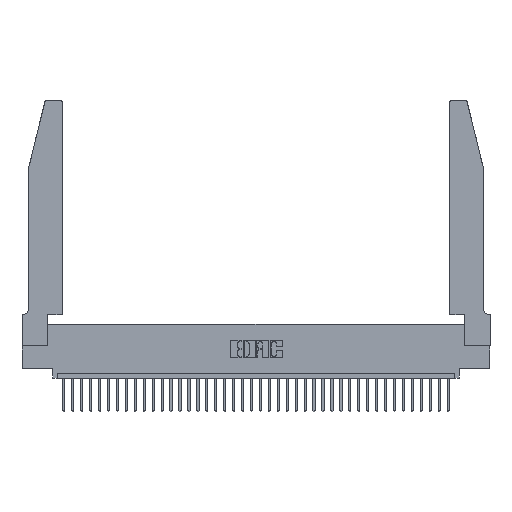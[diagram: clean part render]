
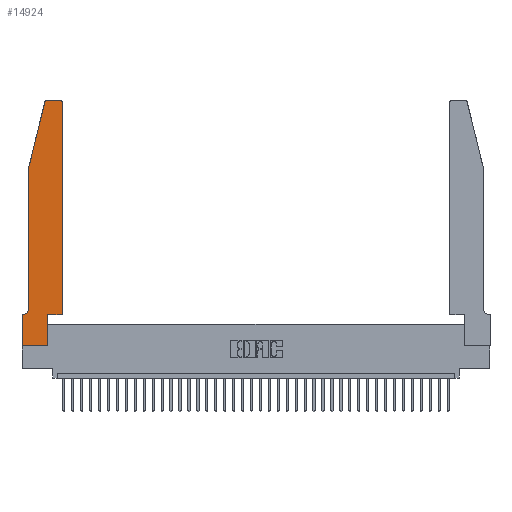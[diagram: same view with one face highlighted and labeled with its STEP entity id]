
A CAD part, top view. The second image highlights one B-rep face of the part: STEP entity #14924.
In plain terms, the highlighted planar face has unit normal (0, 0, 1).
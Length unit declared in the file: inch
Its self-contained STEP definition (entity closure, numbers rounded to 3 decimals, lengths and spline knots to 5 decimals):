
#1022 = ORIENTED_EDGE ( 'NONE', *, *, #9327, .T. ) ;
#1280 = AXIS2_PLACEMENT_3D ( 'NONE', #3978, #37201, #30963 ) ;
#2041 = LINE ( 'NONE', #30785, #21114 ) ;
#2487 = DIRECTION ( 'NONE',  ( -1., 0., 0. ) ) ;
#2624 = CARTESIAN_POINT ( 'NONE',  ( 0.284, 2.75, 0.37 ) ) ;
#2800 = DIRECTION ( 'NONE',  ( 1., 0., 0. ) ) ;
#3412 = CARTESIAN_POINT ( 'NONE',  ( 0.4505, 0.35, 0.37 ) ) ;
#3474 = AXIS2_PLACEMENT_3D ( 'NONE', #17169, #36990, #7970 ) ;
#3978 = CARTESIAN_POINT ( 'NONE',  ( 0.284, 2.72, 0.37 ) ) ;
#4354 = CARTESIAN_POINT ( 'NONE',  ( 0.4505, 0.35, 0.37 ) ) ;
#4564 = VERTEX_POINT ( 'NONE', #9132 ) ;
#4585 = ORIENTED_EDGE ( 'NONE', *, *, #28018, .T. ) ;
#5076 = DIRECTION ( 'NONE',  ( 0., -1., 0. ) ) ;
#5438 = EDGE_CURVE ( 'NONE', #6268, #27754, #9279, .T. ) ;
#5701 = EDGE_CURVE ( 'NONE', #22428, #12500, #17508, .T. ) ;
#5960 = VERTEX_POINT ( 'NONE', #11096 ) ;
#6268 = VERTEX_POINT ( 'NONE', #3412 ) ;
#6468 = ORIENTED_EDGE ( 'NONE', *, *, #10294, .T. ) ;
#6600 = FACE_OUTER_BOUND ( 'NONE', #17381, .T. ) ;
#7970 = DIRECTION ( 'NONE',  ( -1., 0., 0. ) ) ;
#8571 = CARTESIAN_POINT ( 'NONE',  ( 0.0755, 2., 0.37 ) ) ;
#9116 = ORIENTED_EDGE ( 'NONE', *, *, #17537, .T. ) ;
#9132 = CARTESIAN_POINT ( 'NONE',  ( 0., 0., 0.37 ) ) ;
#9237 = EDGE_CURVE ( 'NONE', #11214, #31411, #37270, .T. ) ;
#9279 = LINE ( 'NONE', #15624, #18861 ) ;
#9287 = CARTESIAN_POINT ( 'NONE',  ( 0.0755, 2., 0.37 ) ) ;
#9327 = EDGE_CURVE ( 'NONE', #28320, #5960, #31320, .T. ) ;
#9758 = ORIENTED_EDGE ( 'NONE', *, *, #14775, .T. ) ;
#9852 = DIRECTION ( 'NONE',  ( 1., 0., 0. ) ) ;
#10294 = EDGE_CURVE ( 'NONE', #12500, #27228, #20772, .T. ) ;
#11096 = CARTESIAN_POINT ( 'NONE',  ( 0.2865, 0.35, 0.37 ) ) ;
#11214 = VERTEX_POINT ( 'NONE', #2624 ) ;
#11242 = DIRECTION ( 'NONE',  ( 0., 1., 0. ) ) ;
#11461 = VECTOR ( 'NONE', #37497, 39.37008 ) ;
#12500 = VERTEX_POINT ( 'NONE', #19748 ) ;
#13174 = CARTESIAN_POINT ( 'NONE',  ( 0., 0.35, 0.37 ) ) ;
#13573 = DIRECTION ( 'NONE',  ( -0.239, -0.971, 0. ) ) ;
#13833 = CARTESIAN_POINT ( 'NONE',  ( 0.4505, 2.72, 0.37 ) ) ;
#14086 = CARTESIAN_POINT ( 'NONE',  ( 0.2865, 0.35, 0.37 ) ) ;
#14120 = CARTESIAN_POINT ( 'NONE',  ( 0.0055, 0.35, 0.37 ) ) ;
#14494 = VECTOR ( 'NONE', #11242, 39.37008 ) ;
#14775 = EDGE_CURVE ( 'NONE', #27228, #23643, #18446, .T. ) ;
#14924 = ADVANCED_FACE ( 'NONE', ( #6600 ), #35068, .T. ) ;
#15624 = CARTESIAN_POINT ( 'NONE',  ( 0.4505, 0.35, 0.37 ) ) ;
#16125 = ORIENTED_EDGE ( 'NONE', *, *, #9237, .T. ) ;
#16747 = CIRCLE ( 'NONE', #23662, 0.03 ) ;
#17002 = CARTESIAN_POINT ( 'NONE',  ( 0.2865, 0., 0.37 ) ) ;
#17169 = CARTESIAN_POINT ( 'NONE',  ( 0.0055, 0.42, 0.37 ) ) ;
#17381 = EDGE_LOOP ( 'NONE', ( #22446, #16125, #9116, #26632, #6468, #9758, #4585, #31067, #1022, #33050, #27022, #35075 ) ) ;
#17508 = LINE ( 'NONE', #8571, #27472 ) ;
#17537 = EDGE_CURVE ( 'NONE', #31411, #22428, #23855, .T. ) ;
#18264 = DIRECTION ( 'NONE',  ( 0., 1., 0. ) ) ;
#18343 = VECTOR ( 'NONE', #2487, 39.37008 ) ;
#18446 = LINE ( 'NONE', #22811, #29827 ) ;
#18861 = VECTOR ( 'NONE', #18264, 39.37008 ) ;
#19184 = LINE ( 'NONE', #19906, #11461 ) ;
#19748 = CARTESIAN_POINT ( 'NONE',  ( 0.0755, 0.42, 0.37 ) ) ;
#19776 = LINE ( 'NONE', #37239, #18343 ) ;
#19906 = CARTESIAN_POINT ( 'NONE',  ( 0., 0., 0.37 ) ) ;
#20772 = CIRCLE ( 'NONE', #3474, 0.07 ) ;
#21114 = VECTOR ( 'NONE', #5076, 39.37008 ) ;
#22428 = VERTEX_POINT ( 'NONE', #9287 ) ;
#22446 = ORIENTED_EDGE ( 'NONE', *, *, #35502, .T. ) ;
#22638 = CARTESIAN_POINT ( 'NONE',  ( 0.4205, 2.75, 0.37 ) ) ;
#22811 = CARTESIAN_POINT ( 'NONE',  ( 0.0755, 0.35, 0.37 ) ) ;
#23456 = EDGE_CURVE ( 'NONE', #4564, #28320, #19184, .T. ) ;
#23643 = VERTEX_POINT ( 'NONE', #32786 ) ;
#23662 = AXIS2_PLACEMENT_3D ( 'NONE', #33042, #30212, #36486 ) ;
#23855 = LINE ( 'NONE', #35709, #26146 ) ;
#26146 = VECTOR ( 'NONE', #13573, 39.37008 ) ;
#26199 = DIRECTION ( 'NONE',  ( 0., -1., 0. ) ) ;
#26600 = LINE ( 'NONE', #4354, #33493 ) ;
#26632 = ORIENTED_EDGE ( 'NONE', *, *, #5701, .T. ) ;
#27022 = ORIENTED_EDGE ( 'NONE', *, *, #5438, .T. ) ;
#27222 = AXIS2_PLACEMENT_3D ( 'NONE', #13174, #33543, #9852 ) ;
#27228 = VERTEX_POINT ( 'NONE', #14120 ) ;
#27472 = VECTOR ( 'NONE', #26199, 39.37008 ) ;
#27613 = EDGE_CURVE ( 'NONE', #5960, #6268, #26600, .T. ) ;
#27754 = VERTEX_POINT ( 'NONE', #13833 ) ;
#28018 = EDGE_CURVE ( 'NONE', #23643, #4564, #2041, .T. ) ;
#28320 = VERTEX_POINT ( 'NONE', #17002 ) ;
#29192 = VERTEX_POINT ( 'NONE', #22638 ) ;
#29827 = VECTOR ( 'NONE', #36942, 39.37008 ) ;
#30212 = DIRECTION ( 'NONE',  ( 0., 0., 1. ) ) ;
#30785 = CARTESIAN_POINT ( 'NONE',  ( 0., 0., 0.37 ) ) ;
#30963 = DIRECTION ( 'NONE',  ( 1., 0., 0. ) ) ;
#31067 = ORIENTED_EDGE ( 'NONE', *, *, #23456, .T. ) ;
#31320 = LINE ( 'NONE', #14086, #14494 ) ;
#31411 = VERTEX_POINT ( 'NONE', #32960 ) ;
#32786 = CARTESIAN_POINT ( 'NONE',  ( 0., 0.35, 0.37 ) ) ;
#32960 = CARTESIAN_POINT ( 'NONE',  ( 0.25487, 2.72718, 0.37 ) ) ;
#33042 = CARTESIAN_POINT ( 'NONE',  ( 0.4205, 2.72, 0.37 ) ) ;
#33050 = ORIENTED_EDGE ( 'NONE', *, *, #27613, .T. ) ;
#33493 = VECTOR ( 'NONE', #2800, 39.37008 ) ;
#33543 = DIRECTION ( 'NONE',  ( 0., 0., 1. ) ) ;
#35068 = PLANE ( 'NONE',  #27222 ) ;
#35075 = ORIENTED_EDGE ( 'NONE', *, *, #35128, .T. ) ;
#35128 = EDGE_CURVE ( 'NONE', #27754, #29192, #16747, .T. ) ;
#35502 = EDGE_CURVE ( 'NONE', #29192, #11214, #19776, .T. ) ;
#35709 = CARTESIAN_POINT ( 'NONE',  ( 0.0755, 2., 0.37 ) ) ;
#36486 = DIRECTION ( 'NONE',  ( 1., 0., 0. ) ) ;
#36942 = DIRECTION ( 'NONE',  ( -1., 0., 0. ) ) ;
#36990 = DIRECTION ( 'NONE',  ( 0., 0., -1. ) ) ;
#37201 = DIRECTION ( 'NONE',  ( 0., 0., 1. ) ) ;
#37239 = CARTESIAN_POINT ( 'NONE',  ( 0.2605, 2.75, 0.37 ) ) ;
#37270 = CIRCLE ( 'NONE', #1280, 0.03 ) ;
#37497 = DIRECTION ( 'NONE',  ( 1., 0., 0. ) ) ;
